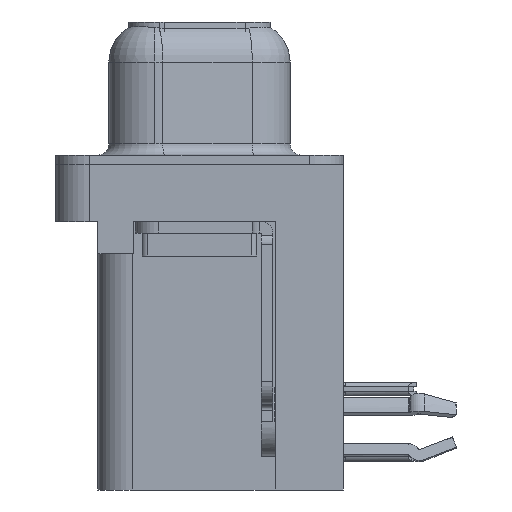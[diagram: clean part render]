
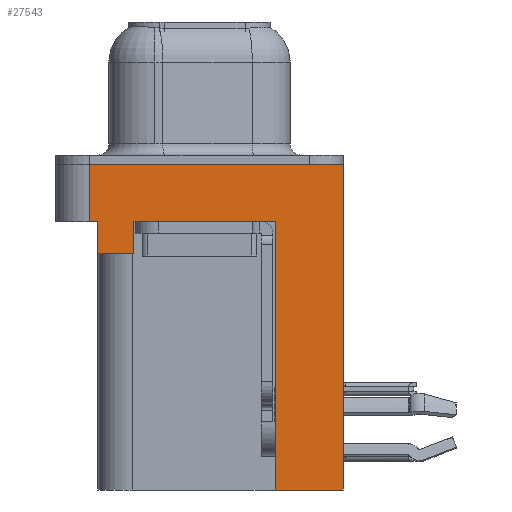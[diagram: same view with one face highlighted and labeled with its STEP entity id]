
A CAD part, left-side view. The second image highlights one B-rep face of the part: STEP entity #27543.
In plain terms, the highlighted planar face has unit normal (-1, 0, 0).
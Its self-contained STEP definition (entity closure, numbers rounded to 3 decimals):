
#985 = CARTESIAN_POINT ( 'NONE',  ( -3., 4.775, -2.5 ) ) ;
#1220 = ORIENTED_EDGE ( 'NONE', *, *, #15942, .F. ) ;
#1404 = EDGE_LOOP ( 'NONE', ( #11703, #5785, #4516, #29046, #14584, #28014, #12313, #6046, #1220, #11620 ) ) ;
#1694 = CARTESIAN_POINT ( 'NONE',  ( -3., -6.275, 0. ) ) ;
#2490 = VERTEX_POINT ( 'NONE', #9720 ) ;
#3634 = EDGE_CURVE ( 'NONE', #9723, #16908, #14489, .T. ) ;
#3670 = EDGE_CURVE ( 'NONE', #2490, #3886, #19564, .T. ) ;
#3764 = VECTOR ( 'NONE', #11690, 1000. ) ;
#3886 = VERTEX_POINT ( 'NONE', #8707 ) ;
#3901 = VECTOR ( 'NONE', #20007, 1000. ) ;
#4319 = CARTESIAN_POINT ( 'NONE',  ( -3., -3.295, -14.2 ) ) ;
#4417 = VERTEX_POINT ( 'NONE', #13925 ) ;
#4516 = ORIENTED_EDGE ( 'NONE', *, *, #12524, .T. ) ;
#5605 = CARTESIAN_POINT ( 'NONE',  ( -3., 2.895, -2.5 ) ) ;
#5785 = ORIENTED_EDGE ( 'NONE', *, *, #18189, .F. ) ;
#5986 = VERTEX_POINT ( 'NONE', #5605 ) ;
#6046 = ORIENTED_EDGE ( 'NONE', *, *, #13302, .F. ) ;
#6655 = DIRECTION ( 'NONE',  ( 0., 0., 1. ) ) ;
#6942 = LINE ( 'NONE', #4319, #15741 ) ;
#6983 = CARTESIAN_POINT ( 'NONE',  ( -3., 4.425, -3.9 ) ) ;
#7485 = VECTOR ( 'NONE', #23169, 1000. ) ;
#8697 = CARTESIAN_POINT ( 'NONE',  ( -3., -6.275, -2.5 ) ) ;
#8707 = CARTESIAN_POINT ( 'NONE',  ( -3., 4.425, -3.9 ) ) ;
#9720 = CARTESIAN_POINT ( 'NONE',  ( -3., 2.895, -3.9 ) ) ;
#9723 = VERTEX_POINT ( 'NONE', #15974 ) ;
#10109 = CARTESIAN_POINT ( 'NONE',  ( -3., -6.275, -2.5 ) ) ;
#10122 = EDGE_CURVE ( 'NONE', #18799, #16908, #23618, .T. ) ;
#10467 = EDGE_CURVE ( 'NONE', #5986, #4417, #24754, .T. ) ;
#10585 = PLANE ( 'NONE',  #14096 ) ;
#10602 = CARTESIAN_POINT ( 'NONE',  ( -3., -6.275, 0. ) ) ;
#10776 = CARTESIAN_POINT ( 'NONE',  ( -3., 2.895, -3.9 ) ) ;
#11620 = ORIENTED_EDGE ( 'NONE', *, *, #10122, .T. ) ;
#11690 = DIRECTION ( 'NONE',  ( 0., -1., 0. ) ) ;
#11703 = ORIENTED_EDGE ( 'NONE', *, *, #3634, .F. ) ;
#12108 = CARTESIAN_POINT ( 'NONE',  ( -3., 4.425, -2.5 ) ) ;
#12297 = DIRECTION ( 'NONE',  ( 0., -1., 0. ) ) ;
#12302 = LINE ( 'NONE', #22948, #3901 ) ;
#12313 = ORIENTED_EDGE ( 'NONE', *, *, #10467, .T. ) ;
#12524 = EDGE_CURVE ( 'NONE', #14879, #23036, #26111, .T. ) ;
#13302 = EDGE_CURVE ( 'NONE', #18889, #4417, #6942, .T. ) ;
#13925 = CARTESIAN_POINT ( 'NONE',  ( -3., -3.295, -2.5 ) ) ;
#14096 = AXIS2_PLACEMENT_3D ( 'NONE', #10109, #20594, #15533 ) ;
#14489 = LINE ( 'NONE', #1694, #3764 ) ;
#14584 = ORIENTED_EDGE ( 'NONE', *, *, #3670, .F. ) ;
#14879 = VERTEX_POINT ( 'NONE', #985 ) ;
#15047 = CARTESIAN_POINT ( 'NONE',  ( -3., -3.295, -14.2 ) ) ;
#15205 = VECTOR ( 'NONE', #30562, 1000. ) ;
#15533 = DIRECTION ( 'NONE',  ( 0., 0., 1. ) ) ;
#15741 = VECTOR ( 'NONE', #29398, 1000. ) ;
#15942 = EDGE_CURVE ( 'NONE', #18799, #18889, #27927, .T. ) ;
#15974 = CARTESIAN_POINT ( 'NONE',  ( -3., 4.775, 0. ) ) ;
#16734 = VECTOR ( 'NONE', #12297, 1000. ) ;
#16908 = VERTEX_POINT ( 'NONE', #10602 ) ;
#18112 = CARTESIAN_POINT ( 'NONE',  ( -3., -6.275, -2.5 ) ) ;
#18189 = EDGE_CURVE ( 'NONE', #14879, #9723, #12302, .T. ) ;
#18688 = VECTOR ( 'NONE', #23989, 1000. ) ;
#18799 = VERTEX_POINT ( 'NONE', #30425 ) ;
#18889 = VERTEX_POINT ( 'NONE', #15047 ) ;
#19564 = LINE ( 'NONE', #26770, #18688 ) ;
#19943 = VECTOR ( 'NONE', #6655, 1000. ) ;
#20007 = DIRECTION ( 'NONE',  ( 0., 0., 1. ) ) ;
#20562 = CARTESIAN_POINT ( 'NONE',  ( -3., -3.295, -14.2 ) ) ;
#20594 = DIRECTION ( 'NONE',  ( -1., 0., 0. ) ) ;
#20779 = LINE ( 'NONE', #10776, #21954 ) ;
#21954 = VECTOR ( 'NONE', #27496, 1000. ) ;
#22948 = CARTESIAN_POINT ( 'NONE',  ( -3., 4.775, -2.5 ) ) ;
#23036 = VERTEX_POINT ( 'NONE', #12108 ) ;
#23169 = DIRECTION ( 'NONE',  ( 0., 1., 0. ) ) ;
#23618 = LINE ( 'NONE', #8697, #25642 ) ;
#23989 = DIRECTION ( 'NONE',  ( 0., 1., 0. ) ) ;
#24754 = LINE ( 'NONE', #29823, #16734 ) ;
#25354 = FACE_OUTER_BOUND ( 'NONE', #1404, .T. ) ;
#25642 = VECTOR ( 'NONE', #30669, 1000. ) ;
#25772 = EDGE_CURVE ( 'NONE', #2490, #5986, #20779, .T. ) ;
#26111 = LINE ( 'NONE', #18112, #15205 ) ;
#26770 = CARTESIAN_POINT ( 'NONE',  ( -3., 4.425, -3.9 ) ) ;
#27496 = DIRECTION ( 'NONE',  ( 0., 0., 1. ) ) ;
#27543 = ADVANCED_FACE ( 'NONE', ( #25354 ), #10585, .T. ) ;
#27927 = LINE ( 'NONE', #20562, #7485 ) ;
#28014 = ORIENTED_EDGE ( 'NONE', *, *, #25772, .T. ) ;
#29046 = ORIENTED_EDGE ( 'NONE', *, *, #29285, .F. ) ;
#29107 = LINE ( 'NONE', #6983, #19943 ) ;
#29285 = EDGE_CURVE ( 'NONE', #3886, #23036, #29107, .T. ) ;
#29398 = DIRECTION ( 'NONE',  ( 0., 0., 1. ) ) ;
#29823 = CARTESIAN_POINT ( 'NONE',  ( -3., -6.275, -2.5 ) ) ;
#30425 = CARTESIAN_POINT ( 'NONE',  ( -3., -6.275, -14.2 ) ) ;
#30562 = DIRECTION ( 'NONE',  ( 0., -1., 0. ) ) ;
#30669 = DIRECTION ( 'NONE',  ( 0., 0., 1. ) ) ;
